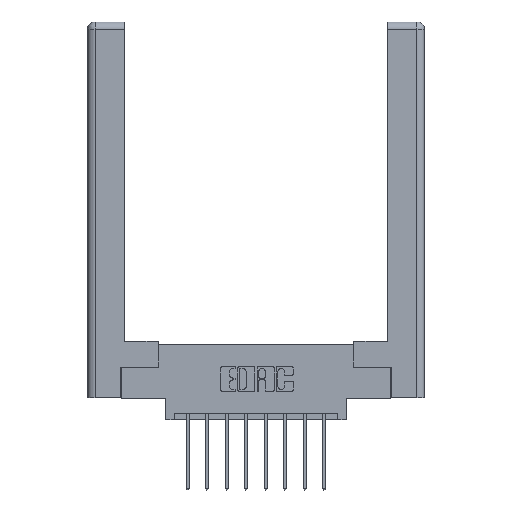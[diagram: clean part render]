
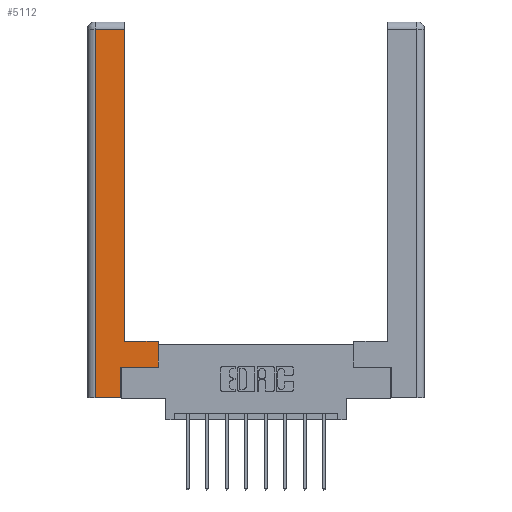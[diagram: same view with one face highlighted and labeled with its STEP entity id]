
A CAD part, top view. The second image highlights one B-rep face of the part: STEP entity #5112.
In plain terms, the highlighted planar face has unit normal (0, 0, 1).
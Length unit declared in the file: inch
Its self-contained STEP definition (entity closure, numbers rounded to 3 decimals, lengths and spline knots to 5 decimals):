
#83 = VERTEX_POINT ( 'NONE', #450 ) ;
#221 = ORIENTED_EDGE ( 'NONE', *, *, #6363, .T. ) ;
#450 = CARTESIAN_POINT ( 'NONE',  ( 0.265, 0., 0. ) ) ;
#510 = CARTESIAN_POINT ( 'NONE',  ( 0.265, 0., 0. ) ) ;
#579 = LINE ( 'NONE', #11746, #8211 ) ;
#660 = ORIENTED_EDGE ( 'NONE', *, *, #3413, .T. ) ;
#688 = DIRECTION ( 'NONE',  ( -1., 0., 0. ) ) ;
#1156 = ORIENTED_EDGE ( 'NONE', *, *, #8928, .T. ) ;
#1399 = CARTESIAN_POINT ( 'NONE',  ( 0.0615, 0., 0. ) ) ;
#1473 = DIRECTION ( 'NONE',  ( 0., 1., 0. ) ) ;
#1571 = AXIS2_PLACEMENT_3D ( 'NONE', #3740, #11970, #688 ) ;
#1841 = CARTESIAN_POINT ( 'NONE',  ( 0.565, 0.245, 0. ) ) ;
#2060 = VECTOR ( 'NONE', #13212, 39.37008 ) ;
#2091 = CARTESIAN_POINT ( 'NONE',  ( 0.0615, 0., 0. ) ) ;
#2160 = LINE ( 'NONE', #8039, #8675 ) ;
#2189 = EDGE_CURVE ( 'NONE', #12093, #9685, #579, .T. ) ;
#2389 = CARTESIAN_POINT ( 'NONE',  ( 0.295, 0.45, 0. ) ) ;
#2539 = LINE ( 'NONE', #2091, #5114 ) ;
#2605 = CARTESIAN_POINT ( 'NONE',  ( 0.565, 0.45, 0. ) ) ;
#2707 = PLANE ( 'NONE',  #1571 ) ;
#3413 = EDGE_CURVE ( 'NONE', #9685, #10345, #7180, .T. ) ;
#3637 = EDGE_LOOP ( 'NONE', ( #7597, #660, #4991, #8965, #221, #12244, #7631, #1156 ) ) ;
#3740 = CARTESIAN_POINT ( 'NONE',  ( 0., 0., 0. ) ) ;
#3856 = LINE ( 'NONE', #1841, #2060 ) ;
#4653 = DIRECTION ( 'NONE',  ( 1., 0., 0. ) ) ;
#4797 = EDGE_CURVE ( 'NONE', #10345, #10227, #2539, .T. ) ;
#4961 = VECTOR ( 'NONE', #4653, 39.37008 ) ;
#4991 = ORIENTED_EDGE ( 'NONE', *, *, #4797, .T. ) ;
#5112 = ADVANCED_FACE ( 'NONE', ( #10460 ), #2707, .F. ) ;
#5114 = VECTOR ( 'NONE', #9297, 39.37008 ) ;
#5190 = VERTEX_POINT ( 'NONE', #9976 ) ;
#5618 = LINE ( 'NONE', #2605, #9167 ) ;
#5680 = LINE ( 'NONE', #6066, #7626 ) ;
#6066 = CARTESIAN_POINT ( 'NONE',  ( 0.295, 0.45, 0. ) ) ;
#6363 = EDGE_CURVE ( 'NONE', #83, #9924, #2160, .T. ) ;
#7180 = LINE ( 'NONE', #12166, #12476 ) ;
#7597 = ORIENTED_EDGE ( 'NONE', *, *, #2189, .T. ) ;
#7626 = VECTOR ( 'NONE', #9061, 39.37008 ) ;
#7631 = ORIENTED_EDGE ( 'NONE', *, *, #12747, .T. ) ;
#7927 = DIRECTION ( 'NONE',  ( 0., 1., 0. ) ) ;
#8039 = CARTESIAN_POINT ( 'NONE',  ( 0.265, 0.245, 0. ) ) ;
#8176 = CARTESIAN_POINT ( 'NONE',  ( 0.295, 2.94, 0. ) ) ;
#8211 = VECTOR ( 'NONE', #1473, 39.37008 ) ;
#8509 = VERTEX_POINT ( 'NONE', #12412 ) ;
#8675 = VECTOR ( 'NONE', #10912, 39.37008 ) ;
#8928 = EDGE_CURVE ( 'NONE', #5190, #12093, #5680, .T. ) ;
#8965 = ORIENTED_EDGE ( 'NONE', *, *, #12187, .T. ) ;
#9061 = DIRECTION ( 'NONE',  ( -1., 0., 0. ) ) ;
#9167 = VECTOR ( 'NONE', #7927, 39.37008 ) ;
#9297 = DIRECTION ( 'NONE',  ( 0., -1., 0. ) ) ;
#9663 = EDGE_CURVE ( 'NONE', #9924, #8509, #3856, .T. ) ;
#9685 = VERTEX_POINT ( 'NONE', #8176 ) ;
#9924 = VERTEX_POINT ( 'NONE', #10409 ) ;
#9976 = CARTESIAN_POINT ( 'NONE',  ( 0.565, 0.45, 0. ) ) ;
#10227 = VERTEX_POINT ( 'NONE', #1399 ) ;
#10242 = DIRECTION ( 'NONE',  ( -1., 0., 0. ) ) ;
#10345 = VERTEX_POINT ( 'NONE', #11001 ) ;
#10409 = CARTESIAN_POINT ( 'NONE',  ( 0.265, 0.245, 0. ) ) ;
#10460 = FACE_OUTER_BOUND ( 'NONE', #3637, .T. ) ;
#10466 = LINE ( 'NONE', #510, #4961 ) ;
#10912 = DIRECTION ( 'NONE',  ( 0., 1., 0. ) ) ;
#11001 = CARTESIAN_POINT ( 'NONE',  ( 0.0615, 2.94, 0. ) ) ;
#11746 = CARTESIAN_POINT ( 'NONE',  ( 0.295, 3., 0. ) ) ;
#11970 = DIRECTION ( 'NONE',  ( 0., 0., -1. ) ) ;
#12093 = VERTEX_POINT ( 'NONE', #2389 ) ;
#12166 = CARTESIAN_POINT ( 'NONE',  ( 0.0615, 2.94, 0. ) ) ;
#12187 = EDGE_CURVE ( 'NONE', #10227, #83, #10466, .T. ) ;
#12244 = ORIENTED_EDGE ( 'NONE', *, *, #9663, .T. ) ;
#12412 = CARTESIAN_POINT ( 'NONE',  ( 0.565, 0.245, 0. ) ) ;
#12476 = VECTOR ( 'NONE', #10242, 39.37008 ) ;
#12747 = EDGE_CURVE ( 'NONE', #8509, #5190, #5618, .T. ) ;
#13212 = DIRECTION ( 'NONE',  ( 1., 0., 0. ) ) ;
